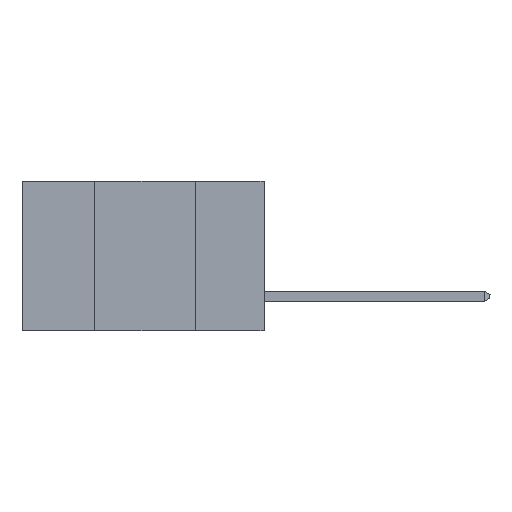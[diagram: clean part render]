
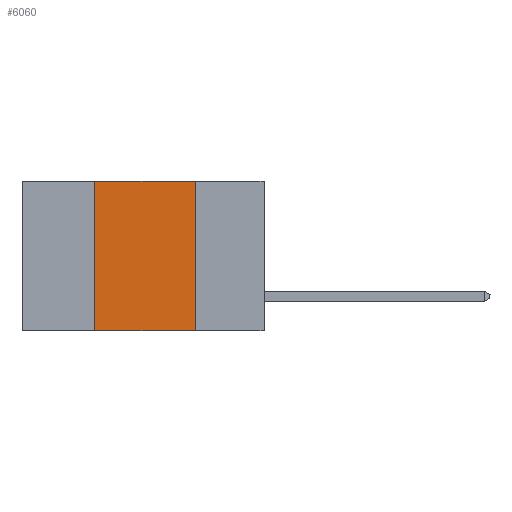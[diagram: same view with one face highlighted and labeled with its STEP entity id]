
A CAD part, left-side view. The second image highlights one B-rep face of the part: STEP entity #6060.
In plain terms, the highlighted planar face has unit normal (-1, 0, 0).
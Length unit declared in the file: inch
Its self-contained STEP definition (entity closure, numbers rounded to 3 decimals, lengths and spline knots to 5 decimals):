
#389 = FACE_OUTER_BOUND ( 'NONE', #8499, .T. ) ;
#439 = VECTOR ( 'NONE', #9750, 39.37008 ) ;
#778 = ORIENTED_EDGE ( 'NONE', *, *, #3168, .F. ) ;
#915 = VECTOR ( 'NONE', #9868, 39.37008 ) ;
#1146 = LINE ( 'NONE', #10095, #6618 ) ;
#1452 = ORIENTED_EDGE ( 'NONE', *, *, #3000, .F. ) ;
#1814 = EDGE_CURVE ( 'NONE', #4359, #9613, #12745, .T. ) ;
#2101 = ORIENTED_EDGE ( 'NONE', *, *, #1814, .T. ) ;
#2374 = DIRECTION ( 'NONE',  ( 0., 0., -1. ) ) ;
#2451 = CARTESIAN_POINT ( 'NONE',  ( 0., 0.17, 0. ) ) ;
#2729 = CARTESIAN_POINT ( 'NONE',  ( 0., 0.6, 0. ) ) ;
#2896 = VERTEX_POINT ( 'NONE', #2451 ) ;
#3000 = EDGE_CURVE ( 'NONE', #10270, #2896, #11016, .T. ) ;
#3168 = EDGE_CURVE ( 'NONE', #4359, #10270, #9207, .T. ) ;
#3931 = DIRECTION ( 'NONE',  ( 0., 0., 1. ) ) ;
#4359 = VERTEX_POINT ( 'NONE', #9996 ) ;
#4753 = DIRECTION ( 'NONE',  ( 1., 0., 0. ) ) ;
#6060 = ADVANCED_FACE ( 'NONE', ( #389 ), #8043, .F. ) ;
#6618 = VECTOR ( 'NONE', #2374, 39.37008 ) ;
#6689 = CARTESIAN_POINT ( 'NONE',  ( 0., 0.6, 0. ) ) ;
#7968 = DIRECTION ( 'NONE',  ( 0., 0., -1. ) ) ;
#8043 = PLANE ( 'NONE',  #13185 ) ;
#8224 = CARTESIAN_POINT ( 'NONE',  ( 0., 0.17, -0.37 ) ) ;
#8292 = CARTESIAN_POINT ( 'NONE',  ( 0., 0.42, 0. ) ) ;
#8499 = EDGE_LOOP ( 'NONE', ( #13797, #1452, #778, #2101 ) ) ;
#9207 = LINE ( 'NONE', #10183, #12498 ) ;
#9279 = CARTESIAN_POINT ( 'NONE',  ( 0., 0.6, -0.37 ) ) ;
#9613 = VERTEX_POINT ( 'NONE', #8224 ) ;
#9679 = EDGE_CURVE ( 'NONE', #2896, #9613, #1146, .T. ) ;
#9750 = DIRECTION ( 'NONE',  ( 0., -1., 0. ) ) ;
#9868 = DIRECTION ( 'NONE',  ( 0., -1., 0. ) ) ;
#9996 = CARTESIAN_POINT ( 'NONE',  ( 0., 0.42, -0.37 ) ) ;
#10095 = CARTESIAN_POINT ( 'NONE',  ( 0., 0.17, -0.37 ) ) ;
#10183 = CARTESIAN_POINT ( 'NONE',  ( 0., 0.42, -0.37 ) ) ;
#10270 = VERTEX_POINT ( 'NONE', #8292 ) ;
#11016 = LINE ( 'NONE', #6689, #915 ) ;
#12498 = VECTOR ( 'NONE', #3931, 39.37008 ) ;
#12745 = LINE ( 'NONE', #9279, #439 ) ;
#13185 = AXIS2_PLACEMENT_3D ( 'NONE', #2729, #4753, #7968 ) ;
#13797 = ORIENTED_EDGE ( 'NONE', *, *, #9679, .F. ) ;
